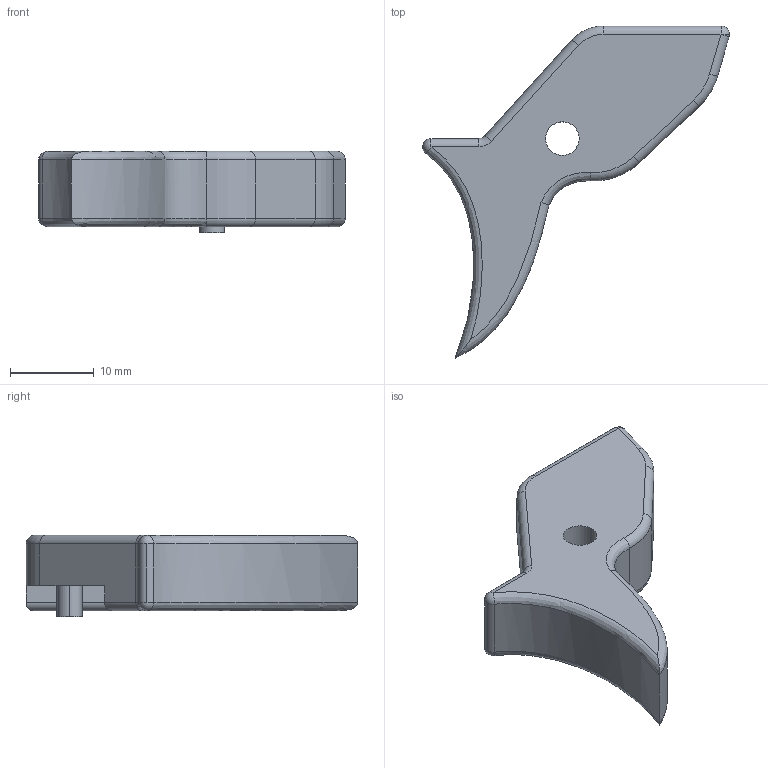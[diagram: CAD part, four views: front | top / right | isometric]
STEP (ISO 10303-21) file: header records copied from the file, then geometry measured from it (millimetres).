
FILE_DESCRIPTION (( 'STEP AP203' ), '1' );
FILE_NAME ('final_trigger.STEP', '2013-07-12T02:42:17', ( '' ), ( '' ), 'SwSTEP 2.0', 'SolidWorks 2012', '' );
FILE_SCHEMA (( 'CONFIG_CONTROL_DESIGN' ));
Length unit declared in the file: millimetre
Products named in the file (1): final_trigger
Bounding box: 36.61 x 39.61 x 9.7 mm (x, y, z)
Volume: 4500.2 mm3; surface area: 2246.4 mm2
Topology: 1 solids, 1 shells, 56 faces, 128 edges, 71 vertices
Faces by surface type: cylinder 23, plane 11, bspline 9, torus 7, sphere 6
Entity records: 2374 total; most frequent: CARTESIAN_POINT 1096, DIRECTION 256, ORIENTED_EDGE 248, EDGE_CURVE 124, AXIS2_PLACEMENT_3D 103, VERTEX_POINT 71, EDGE_LOOP 59, FACE_OUTER_BOUND 56
